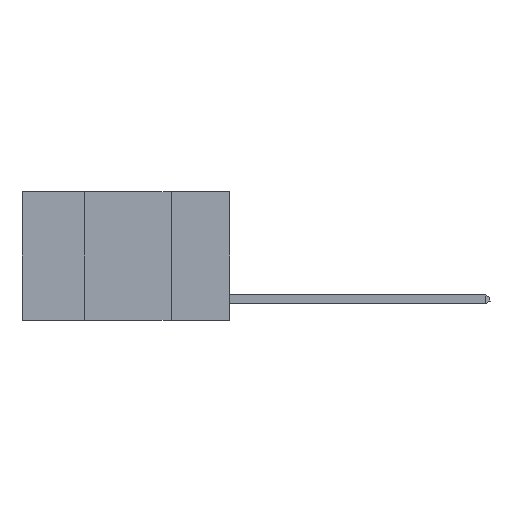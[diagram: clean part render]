
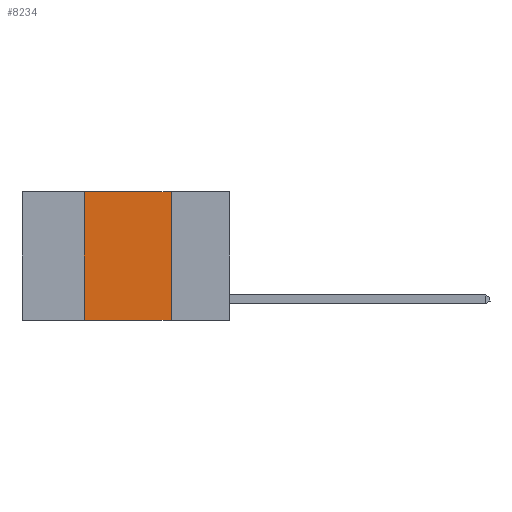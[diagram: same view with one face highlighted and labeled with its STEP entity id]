
A CAD part, left-side view. The second image highlights one B-rep face of the part: STEP entity #8234.
In plain terms, the highlighted planar face has unit normal (-1, 0, 0).
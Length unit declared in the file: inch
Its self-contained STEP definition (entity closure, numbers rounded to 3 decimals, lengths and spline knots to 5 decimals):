
#80 = EDGE_CURVE ( 'NONE', #7273, #18706, #18967, .T. ) ;
#663 = LINE ( 'NONE', #1531, #8097 ) ;
#795 = EDGE_CURVE ( 'NONE', #7273, #12041, #12915, .T. ) ;
#1531 = CARTESIAN_POINT ( 'NONE',  ( 0., 0.6, 0. ) ) ;
#1775 = LINE ( 'NONE', #11022, #9194 ) ;
#2548 = EDGE_CURVE ( 'NONE', #3156, #12041, #1775, .T. ) ;
#3156 = VERTEX_POINT ( 'NONE', #3428 ) ;
#3226 = VECTOR ( 'NONE', #7194, 39.37008 ) ;
#3428 = CARTESIAN_POINT ( 'NONE',  ( 0., 0.17, 0. ) ) ;
#4535 = CARTESIAN_POINT ( 'NONE',  ( 0., 0.6, -0.37 ) ) ;
#6244 = DIRECTION ( 'NONE',  ( 1., 0., 0. ) ) ;
#7194 = DIRECTION ( 'NONE',  ( 0., 0., 1. ) ) ;
#7273 = VERTEX_POINT ( 'NONE', #7344 ) ;
#7344 = CARTESIAN_POINT ( 'NONE',  ( 0., 0.42, -0.37 ) ) ;
#7418 = CARTESIAN_POINT ( 'NONE',  ( 0., 0.42, 0. ) ) ;
#7984 = CARTESIAN_POINT ( 'NONE',  ( 0., 0.42, 0. ) ) ;
#8097 = VECTOR ( 'NONE', #11887, 39.37008 ) ;
#8129 = DIRECTION ( 'NONE',  ( 0., 0., -1. ) ) ;
#8234 = ADVANCED_FACE ( 'NONE', ( #11353 ), #15106, .F. ) ;
#8738 = ORIENTED_EDGE ( 'NONE', *, *, #17844, .F. ) ;
#9194 = VECTOR ( 'NONE', #8129, 39.37008 ) ;
#9895 = ORIENTED_EDGE ( 'NONE', *, *, #795, .T. ) ;
#11022 = CARTESIAN_POINT ( 'NONE',  ( 0., 0.17, 0. ) ) ;
#11353 = FACE_OUTER_BOUND ( 'NONE', #18716, .T. ) ;
#11887 = DIRECTION ( 'NONE',  ( 0., -1., 0. ) ) ;
#12041 = VERTEX_POINT ( 'NONE', #13014 ) ;
#12134 = CARTESIAN_POINT ( 'NONE',  ( 0., 0.6, 0. ) ) ;
#12405 = ORIENTED_EDGE ( 'NONE', *, *, #2548, .F. ) ;
#12915 = LINE ( 'NONE', #4535, #16837 ) ;
#13014 = CARTESIAN_POINT ( 'NONE',  ( 0., 0.17, -0.37 ) ) ;
#13150 = AXIS2_PLACEMENT_3D ( 'NONE', #12134, #6244, #16558 ) ;
#14985 = ORIENTED_EDGE ( 'NONE', *, *, #80, .F. ) ;
#15106 = PLANE ( 'NONE',  #13150 ) ;
#16287 = DIRECTION ( 'NONE',  ( 0., -1., 0. ) ) ;
#16558 = DIRECTION ( 'NONE',  ( 0., 0., -1. ) ) ;
#16837 = VECTOR ( 'NONE', #16287, 39.37008 ) ;
#17844 = EDGE_CURVE ( 'NONE', #18706, #3156, #663, .T. ) ;
#18706 = VERTEX_POINT ( 'NONE', #7984 ) ;
#18716 = EDGE_LOOP ( 'NONE', ( #12405, #8738, #14985, #9895 ) ) ;
#18967 = LINE ( 'NONE', #7418, #3226 ) ;
